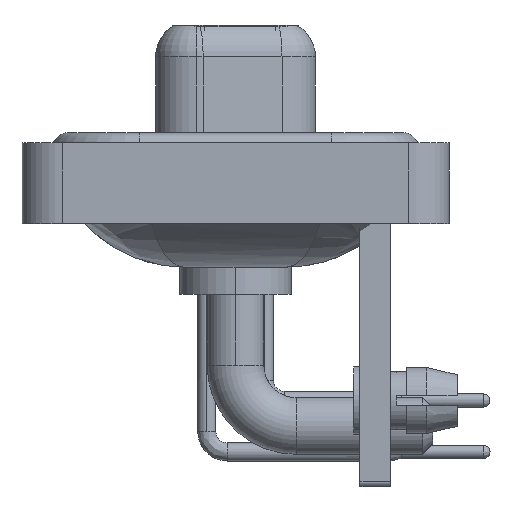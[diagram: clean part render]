
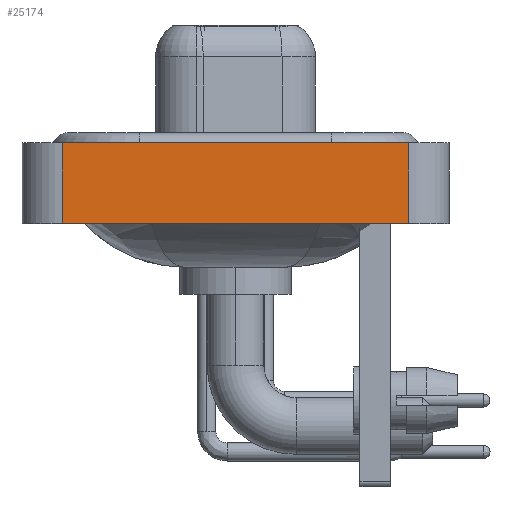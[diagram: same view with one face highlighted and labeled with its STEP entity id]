
A CAD part, left-side view. The second image highlights one B-rep face of the part: STEP entity #25174.
In plain terms, the highlighted planar face has unit normal (-1, 0, 0).
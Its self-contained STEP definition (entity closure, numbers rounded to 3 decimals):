
#8 = CARTESIAN_POINT ( 'NONE',  ( -7.35, -8.55, 0.4 ) ) ;
#448 = CARTESIAN_POINT ( 'NONE',  ( -7.35, -8.55, -3.6 ) ) ;
#2933 = EDGE_CURVE ( 'NONE', #9493, #3172, #5918, .T. ) ;
#3172 = VERTEX_POINT ( 'NONE', #448 ) ;
#3457 = VECTOR ( 'NONE', #3864, 1000. ) ;
#3864 = DIRECTION ( 'NONE',  ( 0., 0., 1. ) ) ;
#3951 = PLANE ( 'NONE',  #6116 ) ;
#5351 = ORIENTED_EDGE ( 'NONE', *, *, #2933, .T. ) ;
#5918 = LINE ( 'NONE', #6180, #26416 ) ;
#6116 = AXIS2_PLACEMENT_3D ( 'NONE', #18727, #16666, #10096 ) ;
#6180 = CARTESIAN_POINT ( 'NONE',  ( -7.35, -8.55, -3.6 ) ) ;
#7499 = CARTESIAN_POINT ( 'NONE',  ( -7.35, 8.55, -3.6 ) ) ;
#7911 = FACE_OUTER_BOUND ( 'NONE', #13203, .T. ) ;
#8214 = VECTOR ( 'NONE', #17621, 1000. ) ;
#8870 = VERTEX_POINT ( 'NONE', #19958 ) ;
#8928 = EDGE_CURVE ( 'NONE', #9493, #25585, #9262, .T. ) ;
#9262 = LINE ( 'NONE', #7499, #8214 ) ;
#9493 = VERTEX_POINT ( 'NONE', #10833 ) ;
#10096 = DIRECTION ( 'NONE',  ( 0., 0., 1. ) ) ;
#10280 = VECTOR ( 'NONE', #19179, 1000. ) ;
#10833 = CARTESIAN_POINT ( 'NONE',  ( -7.35, 8.55, -3.6 ) ) ;
#13203 = EDGE_LOOP ( 'NONE', ( #18993, #24702, #20815, #5351 ) ) ;
#13707 = EDGE_CURVE ( 'NONE', #25585, #8870, #25192, .T. ) ;
#14394 = LINE ( 'NONE', #16859, #3457 ) ;
#16666 = DIRECTION ( 'NONE',  ( -1., 0., 0. ) ) ;
#16859 = CARTESIAN_POINT ( 'NONE',  ( -7.35, -8.55, -3.6 ) ) ;
#17621 = DIRECTION ( 'NONE',  ( 0., 0., 1. ) ) ;
#18373 = DIRECTION ( 'NONE',  ( 0., -1., 0. ) ) ;
#18727 = CARTESIAN_POINT ( 'NONE',  ( -7.35, -8.55, -3.6 ) ) ;
#18993 = ORIENTED_EDGE ( 'NONE', *, *, #22996, .T. ) ;
#19179 = DIRECTION ( 'NONE',  ( 0., -1., 0. ) ) ;
#19958 = CARTESIAN_POINT ( 'NONE',  ( -7.35, -8.55, 0.4 ) ) ;
#20815 = ORIENTED_EDGE ( 'NONE', *, *, #8928, .F. ) ;
#22525 = CARTESIAN_POINT ( 'NONE',  ( -7.35, 8.55, 0.4 ) ) ;
#22996 = EDGE_CURVE ( 'NONE', #3172, #8870, #14394, .T. ) ;
#24702 = ORIENTED_EDGE ( 'NONE', *, *, #13707, .F. ) ;
#25174 = ADVANCED_FACE ( 'NONE', ( #7911 ), #3951, .T. ) ;
#25192 = LINE ( 'NONE', #8, #10280 ) ;
#25585 = VERTEX_POINT ( 'NONE', #22525 ) ;
#26416 = VECTOR ( 'NONE', #18373, 1000. ) ;
